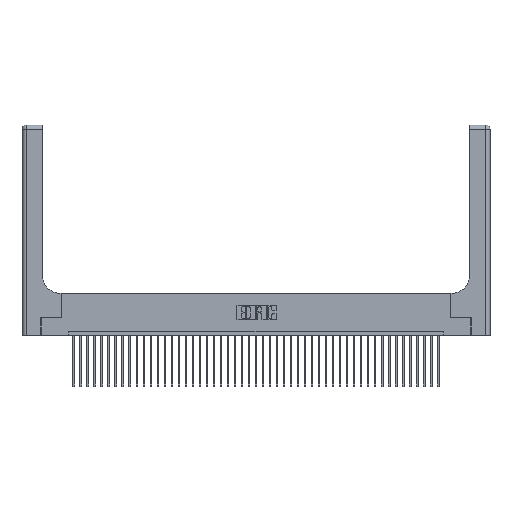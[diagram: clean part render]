
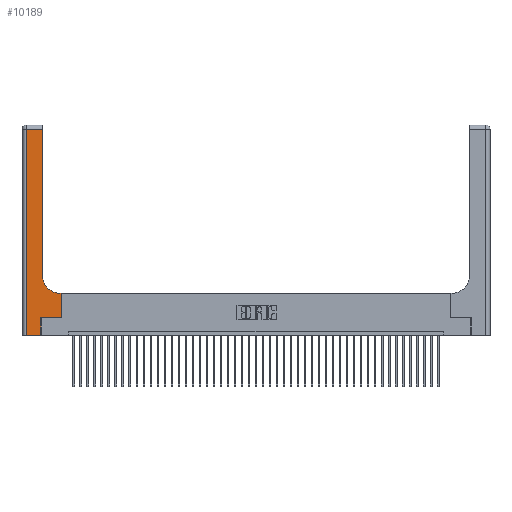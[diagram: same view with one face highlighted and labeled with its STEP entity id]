
A CAD part, top view. The second image highlights one B-rep face of the part: STEP entity #10189.
In plain terms, the highlighted planar face has unit normal (0, 0, 1).
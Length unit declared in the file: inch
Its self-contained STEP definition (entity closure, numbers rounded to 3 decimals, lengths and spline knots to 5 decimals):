
#158 = CARTESIAN_POINT ( 'NONE',  ( 0.5585, 0.25, 0.37 ) ) ;
#580 = DIRECTION ( 'NONE',  ( 0., 1., 0. ) ) ;
#740 = ORIENTED_EDGE ( 'NONE', *, *, #25357, .T. ) ;
#1615 = CARTESIAN_POINT ( 'NONE',  ( 0.5415, 0.85, 0.37 ) ) ;
#1999 = CARTESIAN_POINT ( 'NONE',  ( 0.269, 0., 0.37 ) ) ;
#3173 = DIRECTION ( 'NONE',  ( -1., 0., 0. ) ) ;
#4071 = VECTOR ( 'NONE', #3173, 39.37008 ) ;
#4220 = CARTESIAN_POINT ( 'NONE',  ( 0.2915, 0.85, 0.37 ) ) ;
#4724 = DIRECTION ( 'NONE',  ( -1., 0., 0. ) ) ;
#4727 = DIRECTION ( 'NONE',  ( 0., -1., 0. ) ) ;
#5133 = DIRECTION ( 'NONE',  ( 0., 0., -1. ) ) ;
#5710 = VECTOR ( 'NONE', #580, 39.37008 ) ;
#6211 = LINE ( 'NONE', #31311, #5710 ) ;
#6639 = VECTOR ( 'NONE', #4727, 39.37008 ) ;
#6714 = CARTESIAN_POINT ( 'NONE',  ( 0.269, 0.25, 0.37 ) ) ;
#7070 = ORIENTED_EDGE ( 'NONE', *, *, #16024, .T. ) ;
#8790 = ORIENTED_EDGE ( 'NONE', *, *, #41995, .T. ) ;
#8930 = CARTESIAN_POINT ( 'NONE',  ( 0.2915, 2.94, 0.37 ) ) ;
#10057 = CARTESIAN_POINT ( 'NONE',  ( 0.2915, 0.6, 0.37 ) ) ;
#10189 = ADVANCED_FACE ( 'NONE', ( #13646 ), #30675, .F. ) ;
#11806 = CARTESIAN_POINT ( 'NONE',  ( 0.06, 3., 0.37 ) ) ;
#11879 = VERTEX_POINT ( 'NONE', #21837 ) ;
#12202 = DIRECTION ( 'NONE',  ( 1., 0., 0. ) ) ;
#13378 = DIRECTION ( 'NONE',  ( 0., 1., 0. ) ) ;
#13646 = FACE_OUTER_BOUND ( 'NONE', #25186, .T. ) ;
#14630 = VERTEX_POINT ( 'NONE', #8930 ) ;
#14864 = CARTESIAN_POINT ( 'NONE',  ( 0., 2.94, 0.37 ) ) ;
#15067 = DIRECTION ( 'NONE',  ( -1., 0., 0. ) ) ;
#15082 = DIRECTION ( 'NONE',  ( 1., 0., 0. ) ) ;
#15660 = VERTEX_POINT ( 'NONE', #19155 ) ;
#16024 = EDGE_CURVE ( 'NONE', #11879, #22984, #29780, .T. ) ;
#16471 = AXIS2_PLACEMENT_3D ( 'NONE', #1615, #5133, #28669 ) ;
#17579 = VECTOR ( 'NONE', #15082, 39.37008 ) ;
#18030 = ORIENTED_EDGE ( 'NONE', *, *, #37584, .T. ) ;
#18046 = LINE ( 'NONE', #36455, #34899 ) ;
#19155 = CARTESIAN_POINT ( 'NONE',  ( 0.5585, 0.6, 0.37 ) ) ;
#19279 = EDGE_CURVE ( 'NONE', #14630, #11879, #36363, .T. ) ;
#21303 = VERTEX_POINT ( 'NONE', #4220 ) ;
#21353 = VECTOR ( 'NONE', #40901, 39.37008 ) ;
#21837 = CARTESIAN_POINT ( 'NONE',  ( 0.06, 2.94, 0.37 ) ) ;
#21853 = LINE ( 'NONE', #38920, #17579 ) ;
#22984 = VERTEX_POINT ( 'NONE', #28253 ) ;
#23195 = ORIENTED_EDGE ( 'NONE', *, *, #30778, .T. ) ;
#25108 = DIRECTION ( 'NONE',  ( 0., 0., -1. ) ) ;
#25185 = ORIENTED_EDGE ( 'NONE', *, *, #19279, .T. ) ;
#25186 = EDGE_LOOP ( 'NONE', ( #25279, #25185, #7070, #28990, #740, #23195, #40375, #8790, #18030 ) ) ;
#25279 = ORIENTED_EDGE ( 'NONE', *, *, #33238, .T. ) ;
#25357 = EDGE_CURVE ( 'NONE', #27290, #36105, #18046, .T. ) ;
#25431 = CARTESIAN_POINT ( 'NONE',  ( 0.5415, 0.6, 0.37 ) ) ;
#25979 = LINE ( 'NONE', #29674, #32796 ) ;
#26055 = VERTEX_POINT ( 'NONE', #25431 ) ;
#26221 = LINE ( 'NONE', #10057, #4071 ) ;
#27290 = VERTEX_POINT ( 'NONE', #1999 ) ;
#28253 = CARTESIAN_POINT ( 'NONE',  ( 0.06, 0., 0.37 ) ) ;
#28542 = EDGE_CURVE ( 'NONE', #42136, #15660, #31339, .T. ) ;
#28669 = DIRECTION ( 'NONE',  ( 1., 0., 0. ) ) ;
#28932 = CARTESIAN_POINT ( 'NONE',  ( 0., 3., 0.37 ) ) ;
#28990 = ORIENTED_EDGE ( 'NONE', *, *, #43527, .T. ) ;
#29054 = VECTOR ( 'NONE', #4724, 39.37008 ) ;
#29674 = CARTESIAN_POINT ( 'NONE',  ( 0.269, 0.25, 0.37 ) ) ;
#29780 = LINE ( 'NONE', #11806, #6639 ) ;
#30155 = CIRCLE ( 'NONE', #16471, 0.25 ) ;
#30675 = PLANE ( 'NONE',  #39823 ) ;
#30778 = EDGE_CURVE ( 'NONE', #36105, #42136, #25979, .T. ) ;
#31311 = CARTESIAN_POINT ( 'NONE',  ( 0.2915, 3., 0.37 ) ) ;
#31339 = LINE ( 'NONE', #158, #21353 ) ;
#32796 = VECTOR ( 'NONE', #12202, 39.37008 ) ;
#33238 = EDGE_CURVE ( 'NONE', #21303, #14630, #6211, .T. ) ;
#34899 = VECTOR ( 'NONE', #13378, 39.37008 ) ;
#36105 = VERTEX_POINT ( 'NONE', #6714 ) ;
#36363 = LINE ( 'NONE', #14864, #29054 ) ;
#36455 = CARTESIAN_POINT ( 'NONE',  ( 0.269, 0., 0.37 ) ) ;
#37584 = EDGE_CURVE ( 'NONE', #26055, #21303, #30155, .T. ) ;
#37668 = CARTESIAN_POINT ( 'NONE',  ( 0.5585, 0.25, 0.37 ) ) ;
#38920 = CARTESIAN_POINT ( 'NONE',  ( 0., 0., 0.37 ) ) ;
#39823 = AXIS2_PLACEMENT_3D ( 'NONE', #28932, #25108, #15067 ) ;
#40375 = ORIENTED_EDGE ( 'NONE', *, *, #28542, .T. ) ;
#40901 = DIRECTION ( 'NONE',  ( 0., 1., 0. ) ) ;
#41995 = EDGE_CURVE ( 'NONE', #15660, #26055, #26221, .T. ) ;
#42136 = VERTEX_POINT ( 'NONE', #37668 ) ;
#43527 = EDGE_CURVE ( 'NONE', #22984, #27290, #21853, .T. ) ;
